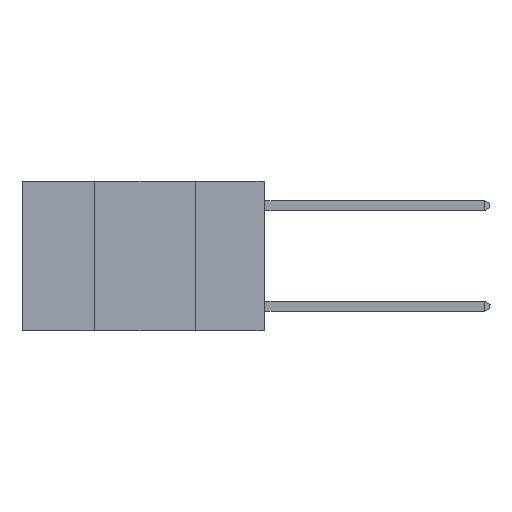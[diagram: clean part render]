
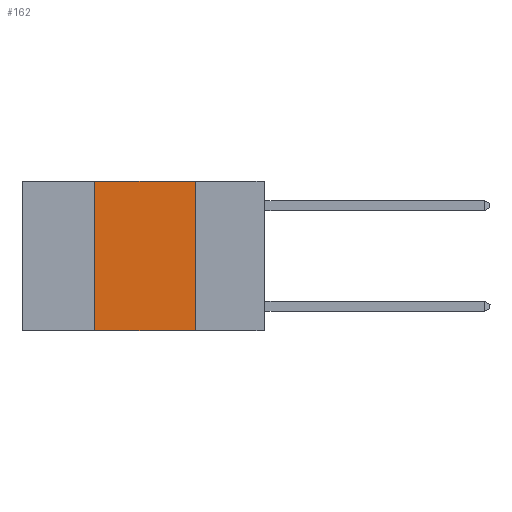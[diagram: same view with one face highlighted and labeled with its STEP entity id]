
A CAD part, left-side view. The second image highlights one B-rep face of the part: STEP entity #162.
In plain terms, the highlighted planar face has unit normal (-1, 0, 0).
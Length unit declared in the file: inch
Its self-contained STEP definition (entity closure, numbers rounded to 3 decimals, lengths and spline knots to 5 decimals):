
#157 = EDGE_CURVE ( 'NONE', #9032, #6563, #8672, .T. ) ;
#162 = ADVANCED_FACE ( 'NONE', ( #8412 ), #10692, .F. ) ;
#240 = VERTEX_POINT ( 'NONE', #8105 ) ;
#685 = CARTESIAN_POINT ( 'NONE',  ( 0., 0.17, 0. ) ) ;
#1285 = EDGE_CURVE ( 'NONE', #240, #7847, #4498, .T. ) ;
#1419 = VECTOR ( 'NONE', #7859, 39.37008 ) ;
#1443 = VECTOR ( 'NONE', #5389, 39.37008 ) ;
#1799 = EDGE_CURVE ( 'NONE', #7847, #6563, #10733, .T. ) ;
#2317 = DIRECTION ( 'NONE',  ( 0., 0., -1. ) ) ;
#2552 = DIRECTION ( 'NONE',  ( 1., 0., 0. ) ) ;
#2754 = AXIS2_PLACEMENT_3D ( 'NONE', #9281, #2552, #2317 ) ;
#3079 = EDGE_LOOP ( 'NONE', ( #8102, #3732, #6064, #8373 ) ) ;
#3732 = ORIENTED_EDGE ( 'NONE', *, *, #1285, .F. ) ;
#4498 = LINE ( 'NONE', #5575, #11134 ) ;
#5180 = DIRECTION ( 'NONE',  ( 0., -1., 0. ) ) ;
#5389 = DIRECTION ( 'NONE',  ( 0., 0., 1. ) ) ;
#5575 = CARTESIAN_POINT ( 'NONE',  ( 0., 0.6, 0. ) ) ;
#5587 = DIRECTION ( 'NONE',  ( 0., -1., 0. ) ) ;
#5624 = LINE ( 'NONE', #11407, #1443 ) ;
#5774 = CARTESIAN_POINT ( 'NONE',  ( 0., 0.42, -0.37 ) ) ;
#6064 = ORIENTED_EDGE ( 'NONE', *, *, #9397, .F. ) ;
#6171 = CARTESIAN_POINT ( 'NONE',  ( 0., 0.6, -0.37 ) ) ;
#6395 = VECTOR ( 'NONE', #5180, 39.37008 ) ;
#6563 = VERTEX_POINT ( 'NONE', #6665 ) ;
#6665 = CARTESIAN_POINT ( 'NONE',  ( 0., 0.17, -0.37 ) ) ;
#7847 = VERTEX_POINT ( 'NONE', #10624 ) ;
#7859 = DIRECTION ( 'NONE',  ( 0., 0., -1. ) ) ;
#8102 = ORIENTED_EDGE ( 'NONE', *, *, #1799, .F. ) ;
#8105 = CARTESIAN_POINT ( 'NONE',  ( 0., 0.42, 0. ) ) ;
#8373 = ORIENTED_EDGE ( 'NONE', *, *, #157, .T. ) ;
#8412 = FACE_OUTER_BOUND ( 'NONE', #3079, .T. ) ;
#8672 = LINE ( 'NONE', #6171, #6395 ) ;
#9032 = VERTEX_POINT ( 'NONE', #5774 ) ;
#9281 = CARTESIAN_POINT ( 'NONE',  ( 0., 0.6, 0. ) ) ;
#9397 = EDGE_CURVE ( 'NONE', #9032, #240, #5624, .T. ) ;
#10624 = CARTESIAN_POINT ( 'NONE',  ( 0., 0.17, 0. ) ) ;
#10692 = PLANE ( 'NONE',  #2754 ) ;
#10733 = LINE ( 'NONE', #685, #1419 ) ;
#11134 = VECTOR ( 'NONE', #5587, 39.37008 ) ;
#11407 = CARTESIAN_POINT ( 'NONE',  ( 0., 0.42, 0. ) ) ;
